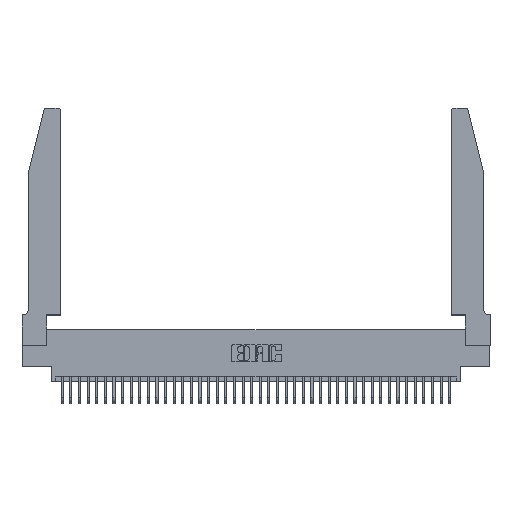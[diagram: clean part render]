
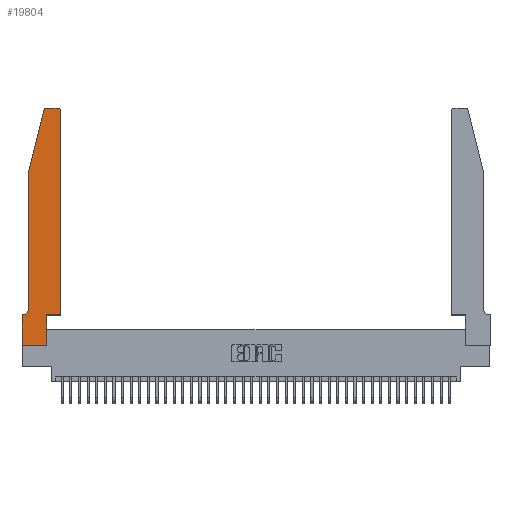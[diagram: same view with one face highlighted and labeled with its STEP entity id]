
A CAD part, top view. The second image highlights one B-rep face of the part: STEP entity #19804.
In plain terms, the highlighted planar face has unit normal (0, 0, 1).
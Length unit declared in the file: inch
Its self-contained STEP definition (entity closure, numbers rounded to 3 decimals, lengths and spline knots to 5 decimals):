
#774 = LINE ( 'NONE', #34112, #38949 ) ;
#1287 = CARTESIAN_POINT ( 'NONE',  ( 0.2865, 0., 0.37 ) ) ;
#2024 = CARTESIAN_POINT ( 'NONE',  ( 0.0755, 2., 0.37 ) ) ;
#2112 = EDGE_CURVE ( 'NONE', #19878, #23826, #14722, .T. ) ;
#2444 = CARTESIAN_POINT ( 'NONE',  ( 0.0055, 0.42, 0.37 ) ) ;
#2544 = VERTEX_POINT ( 'NONE', #35939 ) ;
#2820 = CARTESIAN_POINT ( 'NONE',  ( 0.0755, 0.35, 0.37 ) ) ;
#4056 = DIRECTION ( 'NONE',  ( 1., 0., 0. ) ) ;
#4419 = ORIENTED_EDGE ( 'NONE', *, *, #10880, .T. ) ;
#4746 = PLANE ( 'NONE',  #36055 ) ;
#5301 = VECTOR ( 'NONE', #23943, 39.37008 ) ;
#5343 = EDGE_CURVE ( 'NONE', #27203, #14746, #26265, .T. ) ;
#5519 = DIRECTION ( 'NONE',  ( -1., 0., 0. ) ) ;
#5838 = AXIS2_PLACEMENT_3D ( 'NONE', #30975, #12971, #33977 ) ;
#6059 = ORIENTED_EDGE ( 'NONE', *, *, #5343, .T. ) ;
#6175 = DIRECTION ( 'NONE',  ( -0.239, -0.971, 0. ) ) ;
#7282 = ORIENTED_EDGE ( 'NONE', *, *, #32375, .T. ) ;
#7770 = ORIENTED_EDGE ( 'NONE', *, *, #34751, .T. ) ;
#7962 = DIRECTION ( 'NONE',  ( -1., 0., 0. ) ) ;
#9016 = VECTOR ( 'NONE', #6175, 39.37008 ) ;
#9116 = VERTEX_POINT ( 'NONE', #21049 ) ;
#9889 = LINE ( 'NONE', #17422, #24991 ) ;
#10081 = ORIENTED_EDGE ( 'NONE', *, *, #10409, .T. ) ;
#10409 = EDGE_CURVE ( 'NONE', #23826, #36525, #36397, .T. ) ;
#10880 = EDGE_CURVE ( 'NONE', #25471, #2544, #27443, .T. ) ;
#11130 = CARTESIAN_POINT ( 'NONE',  ( 0.2865, 0.35, 0.37 ) ) ;
#11146 = EDGE_CURVE ( 'NONE', #36525, #13396, #17070, .T. ) ;
#12434 = CARTESIAN_POINT ( 'NONE',  ( 0.4505, 0.35, 0.37 ) ) ;
#12971 = DIRECTION ( 'NONE',  ( 0., 0., 1. ) ) ;
#13056 = CARTESIAN_POINT ( 'NONE',  ( 0.25487, 2.72718, 0.37 ) ) ;
#13396 = VERTEX_POINT ( 'NONE', #2024 ) ;
#13454 = CARTESIAN_POINT ( 'NONE',  ( 0.0755, 0.42, 0.37 ) ) ;
#13883 = DIRECTION ( 'NONE',  ( 1., 0., 0. ) ) ;
#14722 = LINE ( 'NONE', #26038, #31662 ) ;
#14746 = VERTEX_POINT ( 'NONE', #15881 ) ;
#14846 = LINE ( 'NONE', #30153, #37856 ) ;
#14884 = VECTOR ( 'NONE', #15471, 39.37008 ) ;
#15308 = ORIENTED_EDGE ( 'NONE', *, *, #24561, .T. ) ;
#15359 = ORIENTED_EDGE ( 'NONE', *, *, #25048, .T. ) ;
#15471 = DIRECTION ( 'NONE',  ( 1., 0., 0. ) ) ;
#15834 = LINE ( 'NONE', #12434, #14884 ) ;
#15881 = CARTESIAN_POINT ( 'NONE',  ( 0.4505, 2.72, 0.37 ) ) ;
#17070 = LINE ( 'NONE', #24249, #9016 ) ;
#17096 = DIRECTION ( 'NONE',  ( 0., 0., 1. ) ) ;
#17422 = CARTESIAN_POINT ( 'NONE',  ( 0.0755, 2., 0.37 ) ) ;
#17582 = CARTESIAN_POINT ( 'NONE',  ( 0.284, 2.75, 0.37 ) ) ;
#17640 = CARTESIAN_POINT ( 'NONE',  ( 0.4505, 0.35, 0.37 ) ) ;
#17647 = ORIENTED_EDGE ( 'NONE', *, *, #11146, .T. ) ;
#17947 = DIRECTION ( 'NONE',  ( -1., 0., 0. ) ) ;
#18296 = VECTOR ( 'NONE', #35610, 39.37008 ) ;
#19804 = ADVANCED_FACE ( 'NONE', ( #22528 ), #4746, .T. ) ;
#19811 = CARTESIAN_POINT ( 'NONE',  ( 0., 0.35, 0.37 ) ) ;
#19878 = VERTEX_POINT ( 'NONE', #26237 ) ;
#20436 = DIRECTION ( 'NONE',  ( 0., -1., 0. ) ) ;
#21049 = CARTESIAN_POINT ( 'NONE',  ( 0., 0., 0.37 ) ) ;
#21724 = EDGE_CURVE ( 'NONE', #30708, #25471, #35173, .T. ) ;
#22280 = LINE ( 'NONE', #38881, #5301 ) ;
#22528 = FACE_OUTER_BOUND ( 'NONE', #32497, .T. ) ;
#23488 = AXIS2_PLACEMENT_3D ( 'NONE', #2444, #23562, #5519 ) ;
#23562 = DIRECTION ( 'NONE',  ( 0., 0., -1. ) ) ;
#23826 = VERTEX_POINT ( 'NONE', #17582 ) ;
#23930 = AXIS2_PLACEMENT_3D ( 'NONE', #35080, #17096, #38068 ) ;
#23943 = DIRECTION ( 'NONE',  ( 0., 1., 0. ) ) ;
#24249 = CARTESIAN_POINT ( 'NONE',  ( 0.0755, 2., 0.37 ) ) ;
#24561 = EDGE_CURVE ( 'NONE', #35565, #37507, #22280, .T. ) ;
#24991 = VECTOR ( 'NONE', #20436, 39.37008 ) ;
#25048 = EDGE_CURVE ( 'NONE', #14746, #19878, #35409, .T. ) ;
#25471 = VERTEX_POINT ( 'NONE', #34663 ) ;
#25960 = EDGE_CURVE ( 'NONE', #13396, #30708, #9889, .T. ) ;
#26038 = CARTESIAN_POINT ( 'NONE',  ( 0.2605, 2.75, 0.37 ) ) ;
#26237 = CARTESIAN_POINT ( 'NONE',  ( 0.4205, 2.75, 0.37 ) ) ;
#26265 = LINE ( 'NONE', #17640, #18296 ) ;
#27203 = VERTEX_POINT ( 'NONE', #31930 ) ;
#27443 = LINE ( 'NONE', #2820, #34478 ) ;
#30153 = CARTESIAN_POINT ( 'NONE',  ( 0., 0., 0.37 ) ) ;
#30708 = VERTEX_POINT ( 'NONE', #13454 ) ;
#30975 = CARTESIAN_POINT ( 'NONE',  ( 0.284, 2.72, 0.37 ) ) ;
#31662 = VECTOR ( 'NONE', #7962, 39.37008 ) ;
#31906 = DIRECTION ( 'NONE',  ( 0., 0., 1. ) ) ;
#31930 = CARTESIAN_POINT ( 'NONE',  ( 0.4505, 0.35, 0.37 ) ) ;
#32375 = EDGE_CURVE ( 'NONE', #37507, #27203, #15834, .T. ) ;
#32497 = EDGE_LOOP ( 'NONE', ( #35973, #10081, #17647, #38730, #32720, #4419, #7770, #36008, #15308, #7282, #6059, #15359 ) ) ;
#32513 = EDGE_CURVE ( 'NONE', #9116, #35565, #774, .T. ) ;
#32720 = ORIENTED_EDGE ( 'NONE', *, *, #21724, .T. ) ;
#33160 = DIRECTION ( 'NONE',  ( 0., -1., 0. ) ) ;
#33977 = DIRECTION ( 'NONE',  ( 1., 0., 0. ) ) ;
#34112 = CARTESIAN_POINT ( 'NONE',  ( 0., 0., 0.37 ) ) ;
#34478 = VECTOR ( 'NONE', #17947, 39.37008 ) ;
#34663 = CARTESIAN_POINT ( 'NONE',  ( 0.0055, 0.35, 0.37 ) ) ;
#34751 = EDGE_CURVE ( 'NONE', #2544, #9116, #14846, .T. ) ;
#35080 = CARTESIAN_POINT ( 'NONE',  ( 0.4205, 2.72, 0.37 ) ) ;
#35173 = CIRCLE ( 'NONE', #23488, 0.07 ) ;
#35409 = CIRCLE ( 'NONE', #23930, 0.03 ) ;
#35565 = VERTEX_POINT ( 'NONE', #1287 ) ;
#35610 = DIRECTION ( 'NONE',  ( 0., 1., 0. ) ) ;
#35939 = CARTESIAN_POINT ( 'NONE',  ( 0., 0.35, 0.37 ) ) ;
#35973 = ORIENTED_EDGE ( 'NONE', *, *, #2112, .T. ) ;
#36008 = ORIENTED_EDGE ( 'NONE', *, *, #32513, .T. ) ;
#36055 = AXIS2_PLACEMENT_3D ( 'NONE', #19811, #31906, #13883 ) ;
#36397 = CIRCLE ( 'NONE', #5838, 0.03 ) ;
#36525 = VERTEX_POINT ( 'NONE', #13056 ) ;
#37507 = VERTEX_POINT ( 'NONE', #11130 ) ;
#37856 = VECTOR ( 'NONE', #33160, 39.37008 ) ;
#38068 = DIRECTION ( 'NONE',  ( 1., 0., 0. ) ) ;
#38730 = ORIENTED_EDGE ( 'NONE', *, *, #25960, .T. ) ;
#38881 = CARTESIAN_POINT ( 'NONE',  ( 0.2865, 0.35, 0.37 ) ) ;
#38949 = VECTOR ( 'NONE', #4056, 39.37008 ) ;
